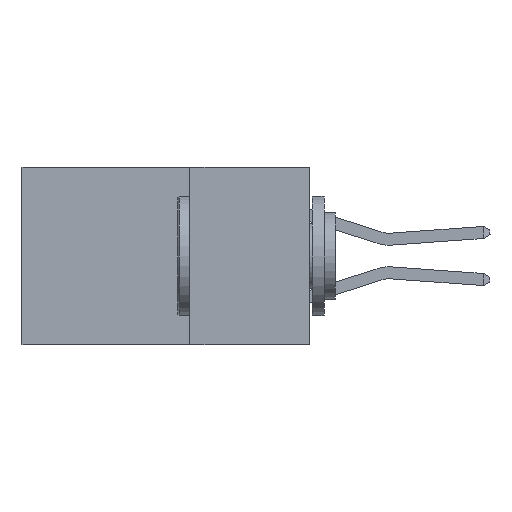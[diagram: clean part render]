
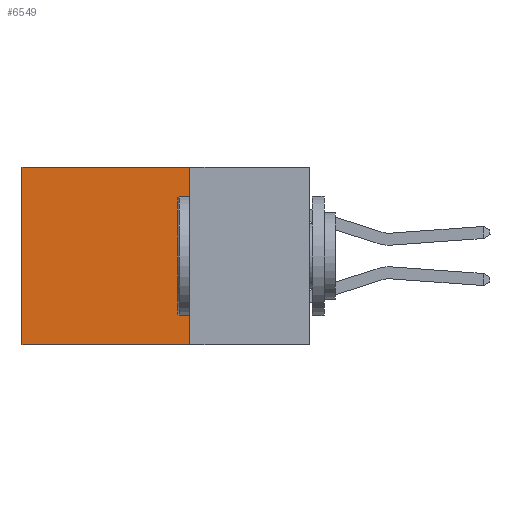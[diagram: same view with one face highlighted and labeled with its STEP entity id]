
A CAD part, left-side view. The second image highlights one B-rep face of the part: STEP entity #6549.
In plain terms, the highlighted planar face has unit normal (-1, 0, 0).
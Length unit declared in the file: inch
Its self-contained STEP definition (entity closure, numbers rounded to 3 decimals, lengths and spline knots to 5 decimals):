
#1087 = DIRECTION ( 'NONE',  ( 0., 1., 0. ) ) ;
#1174 = FACE_OUTER_BOUND ( 'NONE', #9611, .T. ) ;
#1349 = EDGE_CURVE ( 'NONE', #1789, #13583, #2489, .T. ) ;
#1455 = CARTESIAN_POINT ( 'NONE',  ( 0.2615, 0.25, 0. ) ) ;
#1735 = EDGE_CURVE ( 'NONE', #13583, #8190, #9042, .T. ) ;
#1789 = VERTEX_POINT ( 'NONE', #1455 ) ;
#2489 = LINE ( 'NONE', #11387, #12822 ) ;
#2833 = VECTOR ( 'NONE', #1087, 39.37008 ) ;
#3022 = ORIENTED_EDGE ( 'NONE', *, *, #5818, .T. ) ;
#4741 = DIRECTION ( 'NONE',  ( 0., 0., -1. ) ) ;
#4976 = CARTESIAN_POINT ( 'NONE',  ( 0.2615, 0.6, -0.37 ) ) ;
#5147 = EDGE_CURVE ( 'NONE', #1789, #7889, #7941, .T. ) ;
#5818 = EDGE_CURVE ( 'NONE', #7889, #8190, #12618, .T. ) ;
#6444 = DIRECTION ( 'NONE',  ( 0., 0., -1. ) ) ;
#6549 = ADVANCED_FACE ( 'NONE', ( #1174 ), #7940, .F. ) ;
#6621 = VECTOR ( 'NONE', #14008, 39.37008 ) ;
#6853 = DIRECTION ( 'NONE',  ( 0., 1., 0. ) ) ;
#7149 = AXIS2_PLACEMENT_3D ( 'NONE', #10121, #12450, #4741 ) ;
#7819 = CARTESIAN_POINT ( 'NONE',  ( 0.2615, 0.6, -0.37 ) ) ;
#7889 = VERTEX_POINT ( 'NONE', #10074 ) ;
#7940 = PLANE ( 'NONE',  #7149 ) ;
#7941 = LINE ( 'NONE', #13355, #11012 ) ;
#8190 = VERTEX_POINT ( 'NONE', #7819 ) ;
#8631 = CARTESIAN_POINT ( 'NONE',  ( 0.2615, 0.25, -0.37 ) ) ;
#8794 = ORIENTED_EDGE ( 'NONE', *, *, #5147, .T. ) ;
#9042 = LINE ( 'NONE', #13263, #2833 ) ;
#9611 = EDGE_LOOP ( 'NONE', ( #3022, #13614, #12893, #8794 ) ) ;
#10074 = CARTESIAN_POINT ( 'NONE',  ( 0.2615, 0.6, 0. ) ) ;
#10121 = CARTESIAN_POINT ( 'NONE',  ( 0.2615, 0.25, -0.37 ) ) ;
#11012 = VECTOR ( 'NONE', #6853, 39.37008 ) ;
#11387 = CARTESIAN_POINT ( 'NONE',  ( 0.2615, 0.25, -0.37 ) ) ;
#12450 = DIRECTION ( 'NONE',  ( 1., 0., 0. ) ) ;
#12618 = LINE ( 'NONE', #4976, #6621 ) ;
#12822 = VECTOR ( 'NONE', #6444, 39.37008 ) ;
#12893 = ORIENTED_EDGE ( 'NONE', *, *, #1349, .F. ) ;
#13263 = CARTESIAN_POINT ( 'NONE',  ( 0.2615, 0.25, -0.37 ) ) ;
#13355 = CARTESIAN_POINT ( 'NONE',  ( 0.2615, 0.25, 0. ) ) ;
#13583 = VERTEX_POINT ( 'NONE', #8631 ) ;
#13614 = ORIENTED_EDGE ( 'NONE', *, *, #1735, .F. ) ;
#14008 = DIRECTION ( 'NONE',  ( 0., 0., -1. ) ) ;
